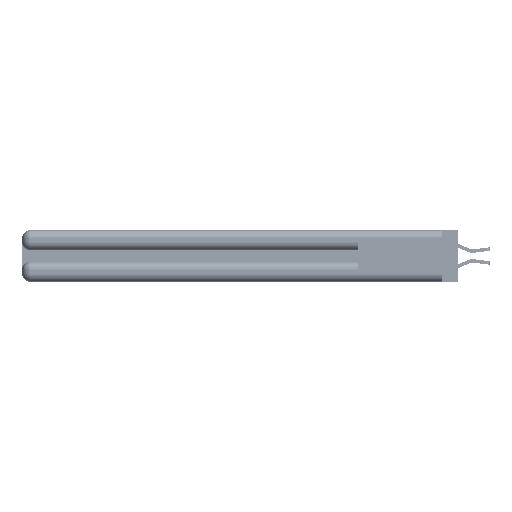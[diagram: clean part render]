
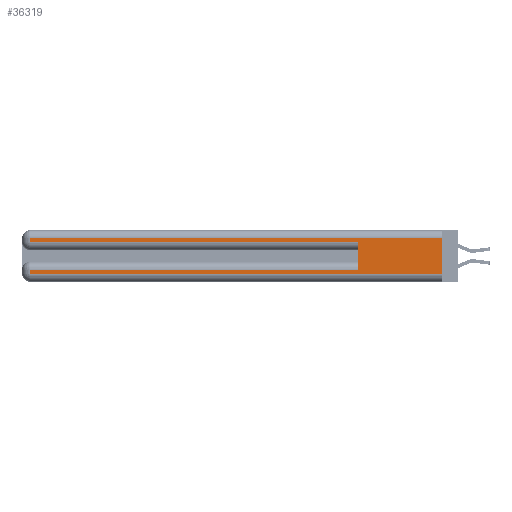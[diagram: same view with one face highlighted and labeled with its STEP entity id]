
A CAD part, left-side view. The second image highlights one B-rep face of the part: STEP entity #36319.
In plain terms, the highlighted planar face has unit normal (-1, 0, 0).
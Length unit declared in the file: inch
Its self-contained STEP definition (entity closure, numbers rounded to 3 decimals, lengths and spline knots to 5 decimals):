
#3131 = CARTESIAN_POINT ( 'NONE',  ( 0., 0., 0.37 ) ) ;
#3560 = LINE ( 'NONE', #31248, #25098 ) ;
#4528 = ORIENTED_EDGE ( 'NONE', *, *, #52149, .T. ) ;
#4850 = DIRECTION ( 'NONE',  ( 0., -1., 0. ) ) ;
#5247 = ORIENTED_EDGE ( 'NONE', *, *, #45966, .T. ) ;
#5293 = CARTESIAN_POINT ( 'NONE',  ( 0., 2.94, 0.31 ) ) ;
#5304 = DIRECTION ( 'NONE',  ( 0., 0., -1. ) ) ;
#6124 = CARTESIAN_POINT ( 'NONE',  ( 0., 2.94, 0.37 ) ) ;
#7051 = EDGE_CURVE ( 'NONE', #36282, #47546, #52882, .T. ) ;
#7438 = DIRECTION ( 'NONE',  ( 1., 0., 0. ) ) ;
#11836 = CARTESIAN_POINT ( 'NONE',  ( 0., 2.94, 0.085 ) ) ;
#17257 = VERTEX_POINT ( 'NONE', #35450 ) ;
#17455 = VERTEX_POINT ( 'NONE', #11836 ) ;
#17742 = CARTESIAN_POINT ( 'NONE',  ( 0., 0., 0.085 ) ) ;
#18444 = EDGE_CURVE ( 'NONE', #32504, #53186, #42628, .T. ) ;
#20816 = CARTESIAN_POINT ( 'NONE',  ( 0., 2.94, 0.37 ) ) ;
#21533 = VECTOR ( 'NONE', #28259, 39.37008 ) ;
#21581 = ORIENTED_EDGE ( 'NONE', *, *, #18444, .F. ) ;
#21815 = EDGE_CURVE ( 'NONE', #32504, #54932, #44261, .T. ) ;
#22993 = CARTESIAN_POINT ( 'NONE',  ( 0., 0., 0.06 ) ) ;
#23748 = VECTOR ( 'NONE', #25115, 39.37008 ) ;
#24135 = CARTESIAN_POINT ( 'NONE',  ( 0., 0.6, 0.145 ) ) ;
#25098 = VECTOR ( 'NONE', #35549, 39.37008 ) ;
#25115 = DIRECTION ( 'NONE',  ( 0., 0., -1. ) ) ;
#25136 = CARTESIAN_POINT ( 'NONE',  ( 0., 0., 0.31 ) ) ;
#25595 = EDGE_LOOP ( 'NONE', ( #21581, #30232, #36913, #27388, #50214, #5247, #4528, #48402 ) ) ;
#26202 = LINE ( 'NONE', #43460, #47577 ) ;
#26740 = EDGE_CURVE ( 'NONE', #30776, #47546, #26202, .T. ) ;
#27388 = ORIENTED_EDGE ( 'NONE', *, *, #26740, .T. ) ;
#27480 = VECTOR ( 'NONE', #37020, 39.37008 ) ;
#28259 = DIRECTION ( 'NONE',  ( 0., 1., 0. ) ) ;
#28860 = PLANE ( 'NONE',  #38156 ) ;
#30232 = ORIENTED_EDGE ( 'NONE', *, *, #21815, .T. ) ;
#30639 = DIRECTION ( 'NONE',  ( 0., 1., 0. ) ) ;
#30776 = VERTEX_POINT ( 'NONE', #54535 ) ;
#31028 = CARTESIAN_POINT ( 'NONE',  ( 0., 0., 0.37 ) ) ;
#31248 = CARTESIAN_POINT ( 'NONE',  ( 0., 0., 0.06 ) ) ;
#31865 = DIRECTION ( 'NONE',  ( 0., 0., -1. ) ) ;
#32504 = VERTEX_POINT ( 'NONE', #25136 ) ;
#33111 = CARTESIAN_POINT ( 'NONE',  ( 0., 0.6, 0.285 ) ) ;
#35450 = CARTESIAN_POINT ( 'NONE',  ( 0., 2.94, 0.06 ) ) ;
#35549 = DIRECTION ( 'NONE',  ( 0., -1., 0. ) ) ;
#36282 = VERTEX_POINT ( 'NONE', #49789 ) ;
#36319 = ADVANCED_FACE ( 'NONE', ( #51932 ), #28860, .F. ) ;
#36913 = ORIENTED_EDGE ( 'NONE', *, *, #38736, .T. ) ;
#37020 = DIRECTION ( 'NONE',  ( 0., 0., 1. ) ) ;
#37316 = EDGE_CURVE ( 'NONE', #17257, #53186, #3560, .T. ) ;
#37474 = DIRECTION ( 'NONE',  ( 0., 0., -1. ) ) ;
#38156 = AXIS2_PLACEMENT_3D ( 'NONE', #3131, #7438, #37474 ) ;
#38736 = EDGE_CURVE ( 'NONE', #54932, #30776, #52438, .T. ) ;
#42395 = VECTOR ( 'NONE', #30639, 39.37008 ) ;
#42628 = LINE ( 'NONE', #31028, #54037 ) ;
#43460 = CARTESIAN_POINT ( 'NONE',  ( 0., 0., 0.285 ) ) ;
#43737 = LINE ( 'NONE', #17742, #42395 ) ;
#44261 = LINE ( 'NONE', #49535, #21533 ) ;
#45966 = EDGE_CURVE ( 'NONE', #36282, #17455, #43737, .T. ) ;
#47546 = VERTEX_POINT ( 'NONE', #33111 ) ;
#47577 = VECTOR ( 'NONE', #4850, 39.37008 ) ;
#47797 = LINE ( 'NONE', #20816, #23748 ) ;
#48402 = ORIENTED_EDGE ( 'NONE', *, *, #37316, .T. ) ;
#49535 = CARTESIAN_POINT ( 'NONE',  ( 0., 0., 0.31 ) ) ;
#49789 = CARTESIAN_POINT ( 'NONE',  ( 0., 0.6, 0.085 ) ) ;
#50214 = ORIENTED_EDGE ( 'NONE', *, *, #7051, .F. ) ;
#51932 = FACE_OUTER_BOUND ( 'NONE', #25595, .T. ) ;
#52149 = EDGE_CURVE ( 'NONE', #17455, #17257, #47797, .T. ) ;
#52438 = LINE ( 'NONE', #6124, #53803 ) ;
#52882 = LINE ( 'NONE', #24135, #27480 ) ;
#53186 = VERTEX_POINT ( 'NONE', #22993 ) ;
#53803 = VECTOR ( 'NONE', #31865, 39.37008 ) ;
#54037 = VECTOR ( 'NONE', #5304, 39.37008 ) ;
#54535 = CARTESIAN_POINT ( 'NONE',  ( 0., 2.94, 0.285 ) ) ;
#54932 = VERTEX_POINT ( 'NONE', #5293 ) ;
